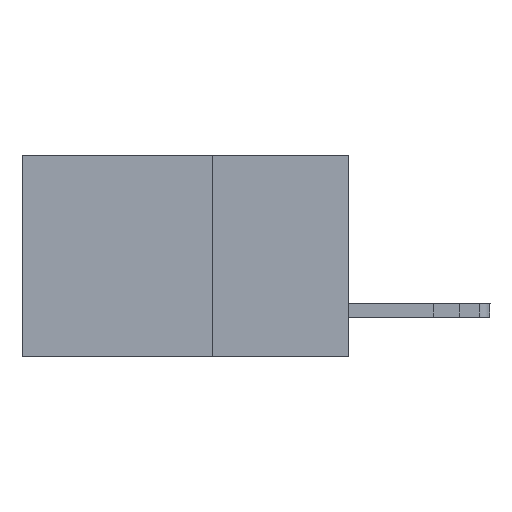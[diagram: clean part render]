
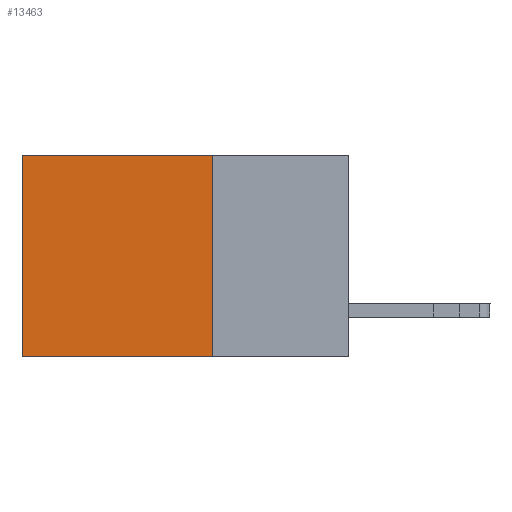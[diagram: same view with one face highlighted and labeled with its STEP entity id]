
A CAD part, left-side view. The second image highlights one B-rep face of the part: STEP entity #13463.
In plain terms, the highlighted planar face has unit normal (-1, 0, 0).
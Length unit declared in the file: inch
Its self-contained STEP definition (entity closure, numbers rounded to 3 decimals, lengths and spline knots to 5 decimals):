
#419 = CARTESIAN_POINT ( 'NONE',  ( 0.2615, 0.6, -0.37 ) ) ;
#439 = VERTEX_POINT ( 'NONE', #20387 ) ;
#1201 = VECTOR ( 'NONE', #16004, 39.37008 ) ;
#1487 = EDGE_CURVE ( 'NONE', #18339, #439, #6769, .T. ) ;
#2093 = DIRECTION ( 'NONE',  ( 0., 0., -1. ) ) ;
#2153 = PLANE ( 'NONE',  #14227 ) ;
#3534 = VECTOR ( 'NONE', #2093, 39.37008 ) ;
#4048 = DIRECTION ( 'NONE',  ( 0., 1., 0. ) ) ;
#5585 = DIRECTION ( 'NONE',  ( 0., 0., -1. ) ) ;
#5691 = CARTESIAN_POINT ( 'NONE',  ( 0.2615, 0.25, 0. ) ) ;
#6769 = LINE ( 'NONE', #5691, #10775 ) ;
#8050 = LINE ( 'NONE', #419, #3534 ) ;
#8094 = ORIENTED_EDGE ( 'NONE', *, *, #8362, .T. ) ;
#8362 = EDGE_CURVE ( 'NONE', #439, #21995, #8050, .T. ) ;
#8531 = VERTEX_POINT ( 'NONE', #14526 ) ;
#9007 = EDGE_CURVE ( 'NONE', #8531, #21995, #19283, .T. ) ;
#9669 = ORIENTED_EDGE ( 'NONE', *, *, #9007, .F. ) ;
#10268 = LINE ( 'NONE', #11838, #18245 ) ;
#10775 = VECTOR ( 'NONE', #4048, 39.37008 ) ;
#11663 = ORIENTED_EDGE ( 'NONE', *, *, #1487, .T. ) ;
#11838 = CARTESIAN_POINT ( 'NONE',  ( 0.2615, 0.25, -0.37 ) ) ;
#12862 = ORIENTED_EDGE ( 'NONE', *, *, #17316, .F. ) ;
#13463 = ADVANCED_FACE ( 'NONE', ( #20935 ), #2153, .F. ) ;
#14082 = CARTESIAN_POINT ( 'NONE',  ( 0.2615, 0.25, -0.37 ) ) ;
#14227 = AXIS2_PLACEMENT_3D ( 'NONE', #14082, #15795, #5585 ) ;
#14526 = CARTESIAN_POINT ( 'NONE',  ( 0.2615, 0.25, -0.37 ) ) ;
#15795 = DIRECTION ( 'NONE',  ( 1., 0., 0. ) ) ;
#16004 = DIRECTION ( 'NONE',  ( 0., 1., 0. ) ) ;
#16911 = DIRECTION ( 'NONE',  ( 0., 0., -1. ) ) ;
#17271 = EDGE_LOOP ( 'NONE', ( #8094, #9669, #12862, #11663 ) ) ;
#17316 = EDGE_CURVE ( 'NONE', #18339, #8531, #10268, .T. ) ;
#18245 = VECTOR ( 'NONE', #16911, 39.37008 ) ;
#18339 = VERTEX_POINT ( 'NONE', #19534 ) ;
#19283 = LINE ( 'NONE', #19421, #1201 ) ;
#19421 = CARTESIAN_POINT ( 'NONE',  ( 0.2615, 0.25, -0.37 ) ) ;
#19534 = CARTESIAN_POINT ( 'NONE',  ( 0.2615, 0.25, 0. ) ) ;
#19833 = CARTESIAN_POINT ( 'NONE',  ( 0.2615, 0.6, -0.37 ) ) ;
#20387 = CARTESIAN_POINT ( 'NONE',  ( 0.2615, 0.6, 0. ) ) ;
#20935 = FACE_OUTER_BOUND ( 'NONE', #17271, .T. ) ;
#21995 = VERTEX_POINT ( 'NONE', #19833 ) ;
